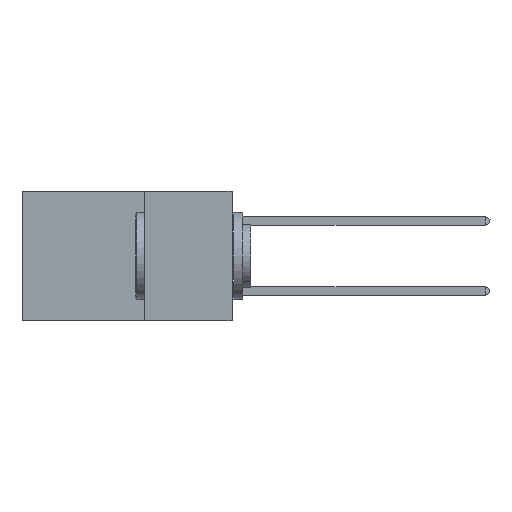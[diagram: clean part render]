
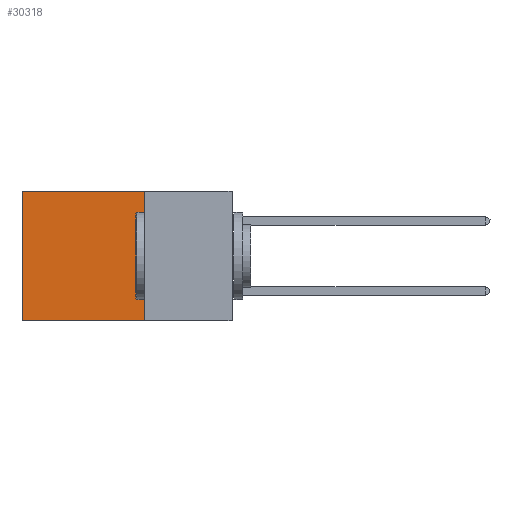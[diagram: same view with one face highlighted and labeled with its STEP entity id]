
A CAD part, left-side view. The second image highlights one B-rep face of the part: STEP entity #30318.
In plain terms, the highlighted planar face has unit normal (-1, 0, 0).
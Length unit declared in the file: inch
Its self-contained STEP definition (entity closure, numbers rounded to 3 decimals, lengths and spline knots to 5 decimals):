
#1021 = VECTOR ( 'NONE', #25242, 39.37008 ) ;
#1572 = VERTEX_POINT ( 'NONE', #9984 ) ;
#2356 = ORIENTED_EDGE ( 'NONE', *, *, #9543, .F. ) ;
#3501 = VECTOR ( 'NONE', #13047, 39.37008 ) ;
#5194 = AXIS2_PLACEMENT_3D ( 'NONE', #31295, #26466, #19078 ) ;
#5710 = CARTESIAN_POINT ( 'NONE',  ( 0.2875, 0.25, 0. ) ) ;
#6216 = EDGE_CURVE ( 'NONE', #18713, #1572, #15444, .T. ) ;
#6835 = VERTEX_POINT ( 'NONE', #7399 ) ;
#7399 = CARTESIAN_POINT ( 'NONE',  ( 0.2875, 0.6, -0.37 ) ) ;
#7457 = FACE_OUTER_BOUND ( 'NONE', #28589, .T. ) ;
#9543 = EDGE_CURVE ( 'NONE', #18713, #17695, #13798, .T. ) ;
#9984 = CARTESIAN_POINT ( 'NONE',  ( 0.2875, 0.6, 0. ) ) ;
#12310 = VECTOR ( 'NONE', #22525, 39.37008 ) ;
#13047 = DIRECTION ( 'NONE',  ( 0., 0., -1. ) ) ;
#13798 = LINE ( 'NONE', #27990, #12310 ) ;
#14233 = VECTOR ( 'NONE', #15835, 39.37008 ) ;
#15444 = LINE ( 'NONE', #5710, #1021 ) ;
#15792 = CARTESIAN_POINT ( 'NONE',  ( 0.2875, 0.6, 0. ) ) ;
#15835 = DIRECTION ( 'NONE',  ( 0., 1., 0. ) ) ;
#16122 = PLANE ( 'NONE',  #5194 ) ;
#16462 = EDGE_CURVE ( 'NONE', #17695, #6835, #19895, .T. ) ;
#17695 = VERTEX_POINT ( 'NONE', #30351 ) ;
#17990 = ORIENTED_EDGE ( 'NONE', *, *, #16462, .F. ) ;
#18713 = VERTEX_POINT ( 'NONE', #24883 ) ;
#19078 = DIRECTION ( 'NONE',  ( 0., 0., -1. ) ) ;
#19895 = LINE ( 'NONE', #25750, #14233 ) ;
#20136 = EDGE_CURVE ( 'NONE', #1572, #6835, #21813, .T. ) ;
#21813 = LINE ( 'NONE', #15792, #3501 ) ;
#22525 = DIRECTION ( 'NONE',  ( 0., 0., -1. ) ) ;
#24883 = CARTESIAN_POINT ( 'NONE',  ( 0.2875, 0.25, 0. ) ) ;
#24897 = ORIENTED_EDGE ( 'NONE', *, *, #6216, .T. ) ;
#25242 = DIRECTION ( 'NONE',  ( 0., 1., 0. ) ) ;
#25750 = CARTESIAN_POINT ( 'NONE',  ( 0.2875, 0.25, -0.37 ) ) ;
#26466 = DIRECTION ( 'NONE',  ( 1., 0., 0. ) ) ;
#27990 = CARTESIAN_POINT ( 'NONE',  ( 0.2875, 0.25, 0. ) ) ;
#28589 = EDGE_LOOP ( 'NONE', ( #30646, #17990, #2356, #24897 ) ) ;
#30318 = ADVANCED_FACE ( 'NONE', ( #7457 ), #16122, .F. ) ;
#30351 = CARTESIAN_POINT ( 'NONE',  ( 0.2875, 0.25, -0.37 ) ) ;
#30646 = ORIENTED_EDGE ( 'NONE', *, *, #20136, .T. ) ;
#31295 = CARTESIAN_POINT ( 'NONE',  ( 0.2875, 0.25, 0. ) ) ;
